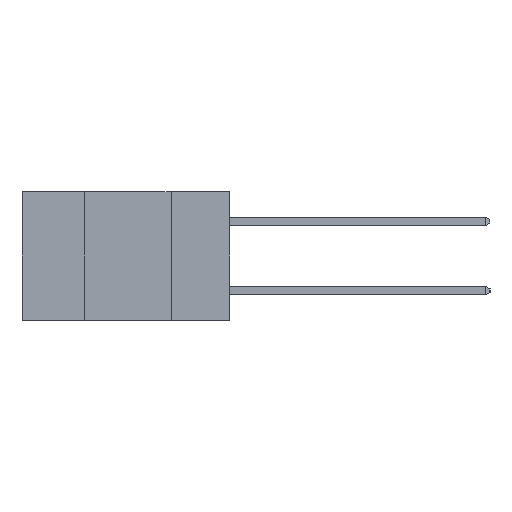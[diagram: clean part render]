
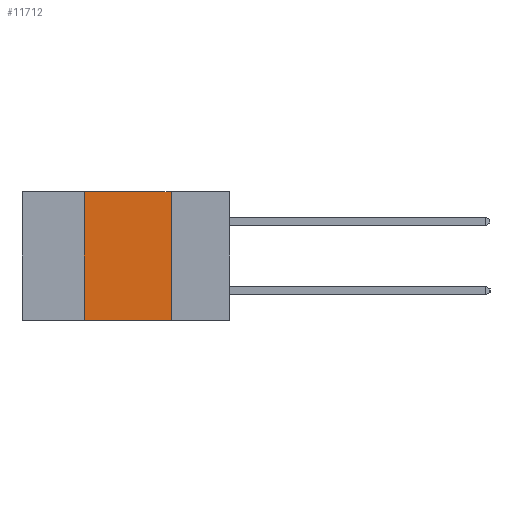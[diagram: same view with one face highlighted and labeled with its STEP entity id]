
A CAD part, left-side view. The second image highlights one B-rep face of the part: STEP entity #11712.
In plain terms, the highlighted planar face has unit normal (-1, 0, 0).
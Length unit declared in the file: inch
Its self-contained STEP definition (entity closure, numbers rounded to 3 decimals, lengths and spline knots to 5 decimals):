
#294 = VECTOR ( 'NONE', #1317, 39.37008 ) ;
#480 = CARTESIAN_POINT ( 'NONE',  ( 0., 0.6, -0.37 ) ) ;
#498 = LINE ( 'NONE', #3038, #4795 ) ;
#1190 = VECTOR ( 'NONE', #7013, 39.37008 ) ;
#1317 = DIRECTION ( 'NONE',  ( 0., 0., 1. ) ) ;
#1388 = EDGE_LOOP ( 'NONE', ( #4357, #11296, #11561, #7014 ) ) ;
#2193 = VERTEX_POINT ( 'NONE', #5891 ) ;
#2807 = PLANE ( 'NONE',  #7978 ) ;
#3038 = CARTESIAN_POINT ( 'NONE',  ( 0., 0.17, -0.37 ) ) ;
#3166 = EDGE_CURVE ( 'NONE', #10951, #6506, #7006, .T. ) ;
#4357 = ORIENTED_EDGE ( 'NONE', *, *, #6373, .F. ) ;
#4437 = VECTOR ( 'NONE', #9550, 39.37008 ) ;
#4684 = DIRECTION ( 'NONE',  ( 0., 0., -1. ) ) ;
#4795 = VECTOR ( 'NONE', #10560, 39.37008 ) ;
#5278 = VERTEX_POINT ( 'NONE', #8696 ) ;
#5891 = CARTESIAN_POINT ( 'NONE',  ( 0., 0.42, -0.37 ) ) ;
#6373 = EDGE_CURVE ( 'NONE', #6506, #5278, #498, .T. ) ;
#6506 = VERTEX_POINT ( 'NONE', #8018 ) ;
#7006 = LINE ( 'NONE', #11432, #4437 ) ;
#7013 = DIRECTION ( 'NONE',  ( 0., -1., 0. ) ) ;
#7014 = ORIENTED_EDGE ( 'NONE', *, *, #8377, .T. ) ;
#7599 = FACE_OUTER_BOUND ( 'NONE', #1388, .T. ) ;
#7867 = CARTESIAN_POINT ( 'NONE',  ( 0., 0.42, -0.37 ) ) ;
#7978 = AXIS2_PLACEMENT_3D ( 'NONE', #9448, #10330, #4684 ) ;
#8018 = CARTESIAN_POINT ( 'NONE',  ( 0., 0.17, 0. ) ) ;
#8377 = EDGE_CURVE ( 'NONE', #2193, #5278, #8966, .T. ) ;
#8696 = CARTESIAN_POINT ( 'NONE',  ( 0., 0.17, -0.37 ) ) ;
#8966 = LINE ( 'NONE', #480, #1190 ) ;
#9387 = EDGE_CURVE ( 'NONE', #2193, #10951, #10206, .T. ) ;
#9448 = CARTESIAN_POINT ( 'NONE',  ( 0., 0.6, 0. ) ) ;
#9550 = DIRECTION ( 'NONE',  ( 0., -1., 0. ) ) ;
#10206 = LINE ( 'NONE', #7867, #294 ) ;
#10251 = CARTESIAN_POINT ( 'NONE',  ( 0., 0.42, 0. ) ) ;
#10330 = DIRECTION ( 'NONE',  ( 1., 0., 0. ) ) ;
#10560 = DIRECTION ( 'NONE',  ( 0., 0., -1. ) ) ;
#10951 = VERTEX_POINT ( 'NONE', #10251 ) ;
#11296 = ORIENTED_EDGE ( 'NONE', *, *, #3166, .F. ) ;
#11432 = CARTESIAN_POINT ( 'NONE',  ( 0., 0.6, 0. ) ) ;
#11561 = ORIENTED_EDGE ( 'NONE', *, *, #9387, .F. ) ;
#11712 = ADVANCED_FACE ( 'NONE', ( #7599 ), #2807, .F. ) ;
